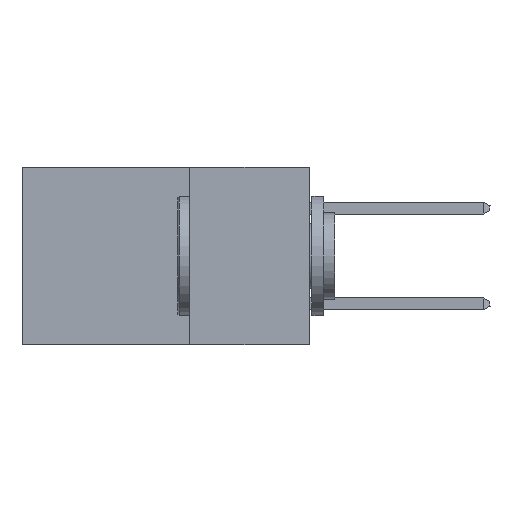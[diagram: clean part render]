
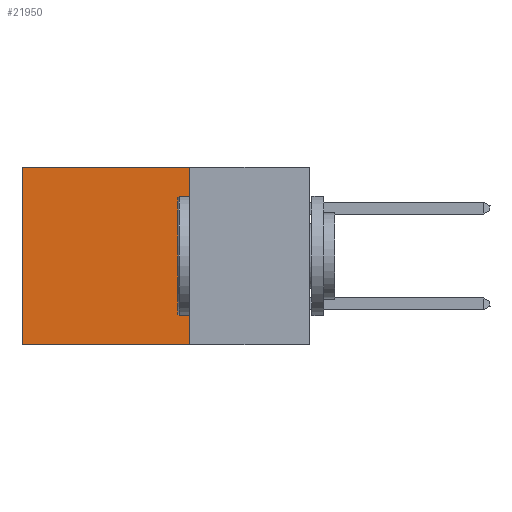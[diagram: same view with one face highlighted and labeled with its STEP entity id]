
A CAD part, left-side view. The second image highlights one B-rep face of the part: STEP entity #21950.
In plain terms, the highlighted planar face has unit normal (-1, 0, 0).
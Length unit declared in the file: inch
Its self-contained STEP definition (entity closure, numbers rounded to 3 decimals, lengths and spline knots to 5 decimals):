
#522 = DIRECTION ( 'NONE',  ( 0., 0., -1. ) ) ;
#1259 = AXIS2_PLACEMENT_3D ( 'NONE', #6414, #17967, #522 ) ;
#1685 = CARTESIAN_POINT ( 'NONE',  ( 0.2875, 0.25, -0.37 ) ) ;
#2217 = ORIENTED_EDGE ( 'NONE', *, *, #24501, .F. ) ;
#3214 = CARTESIAN_POINT ( 'NONE',  ( 0.2875, 0.6, -0.37 ) ) ;
#3362 = CARTESIAN_POINT ( 'NONE',  ( 0.2875, 0.6, 0. ) ) ;
#4176 = CARTESIAN_POINT ( 'NONE',  ( 0.2875, 0.25, 0. ) ) ;
#4843 = VERTEX_POINT ( 'NONE', #1685 ) ;
#5995 = CARTESIAN_POINT ( 'NONE',  ( 0.2875, 0.6, 0. ) ) ;
#6414 = CARTESIAN_POINT ( 'NONE',  ( 0.2875, 0.25, 0. ) ) ;
#6672 = VERTEX_POINT ( 'NONE', #4176 ) ;
#10115 = CARTESIAN_POINT ( 'NONE',  ( 0.2875, 0.25, 0. ) ) ;
#11074 = LINE ( 'NONE', #11249, #26265 ) ;
#11249 = CARTESIAN_POINT ( 'NONE',  ( 0.2875, 0.25, -0.37 ) ) ;
#12591 = LINE ( 'NONE', #34278, #28722 ) ;
#16102 = LINE ( 'NONE', #10115, #30517 ) ;
#17967 = DIRECTION ( 'NONE',  ( 1., 0., 0. ) ) ;
#19507 = EDGE_CURVE ( 'NONE', #23214, #27609, #35137, .T. ) ;
#21950 = ADVANCED_FACE ( 'NONE', ( #24757 ), #26497, .F. ) ;
#22269 = DIRECTION ( 'NONE',  ( 0., 0., -1. ) ) ;
#23214 = VERTEX_POINT ( 'NONE', #5995 ) ;
#24017 = EDGE_LOOP ( 'NONE', ( #34003, #31704, #2217, #32864 ) ) ;
#24501 = EDGE_CURVE ( 'NONE', #6672, #4843, #12591, .T. ) ;
#24757 = FACE_OUTER_BOUND ( 'NONE', #24017, .T. ) ;
#26265 = VECTOR ( 'NONE', #31336, 39.37008 ) ;
#26497 = PLANE ( 'NONE',  #1259 ) ;
#27609 = VERTEX_POINT ( 'NONE', #3214 ) ;
#28722 = VECTOR ( 'NONE', #22269, 39.37008 ) ;
#29887 = EDGE_CURVE ( 'NONE', #6672, #23214, #16102, .T. ) ;
#30517 = VECTOR ( 'NONE', #36002, 39.37008 ) ;
#31336 = DIRECTION ( 'NONE',  ( 0., 1., 0. ) ) ;
#31704 = ORIENTED_EDGE ( 'NONE', *, *, #33847, .F. ) ;
#32864 = ORIENTED_EDGE ( 'NONE', *, *, #29887, .T. ) ;
#33847 = EDGE_CURVE ( 'NONE', #4843, #27609, #11074, .T. ) ;
#34003 = ORIENTED_EDGE ( 'NONE', *, *, #19507, .T. ) ;
#34233 = VECTOR ( 'NONE', #35083, 39.37008 ) ;
#34278 = CARTESIAN_POINT ( 'NONE',  ( 0.2875, 0.25, 0. ) ) ;
#35083 = DIRECTION ( 'NONE',  ( 0., 0., -1. ) ) ;
#35137 = LINE ( 'NONE', #3362, #34233 ) ;
#36002 = DIRECTION ( 'NONE',  ( 0., 1., 0. ) ) ;
